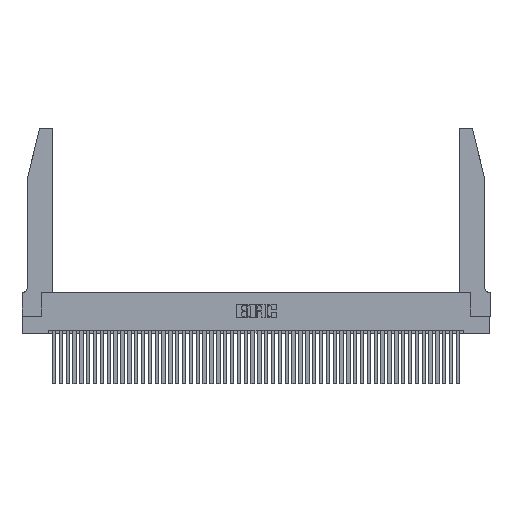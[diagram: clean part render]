
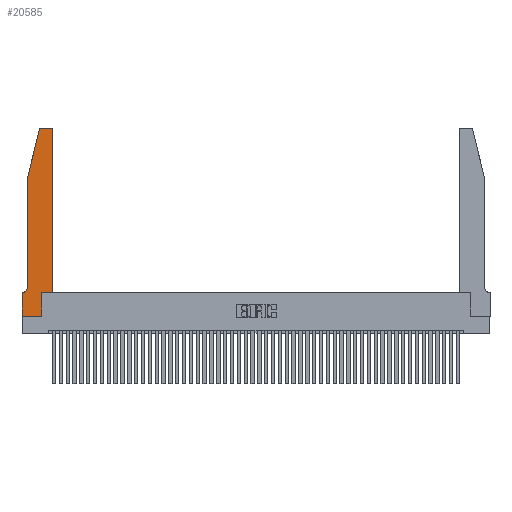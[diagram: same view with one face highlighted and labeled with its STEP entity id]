
A CAD part, top view. The second image highlights one B-rep face of the part: STEP entity #20585.
In plain terms, the highlighted planar face has unit normal (0, 0, 1).
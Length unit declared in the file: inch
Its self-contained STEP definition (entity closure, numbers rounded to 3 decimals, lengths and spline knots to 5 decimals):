
#116 = DIRECTION ( 'NONE',  ( 0., 0., 1. ) ) ;
#883 = CARTESIAN_POINT ( 'NONE',  ( 0.284, 2.72, 0.37 ) ) ;
#1681 = ORIENTED_EDGE ( 'NONE', *, *, #31914, .T. ) ;
#2662 = ORIENTED_EDGE ( 'NONE', *, *, #48983, .T. ) ;
#3055 = VERTEX_POINT ( 'NONE', #15933 ) ;
#3112 = EDGE_CURVE ( 'NONE', #3055, #36527, #25985, .T. ) ;
#3243 = DIRECTION ( 'NONE',  ( 0., 0., 1. ) ) ;
#5115 = CARTESIAN_POINT ( 'NONE',  ( 0.2865, 0.35, 0.37 ) ) ;
#5513 = CARTESIAN_POINT ( 'NONE',  ( 0.2865, 0.35, 0.37 ) ) ;
#5666 = DIRECTION ( 'NONE',  ( -0.239, -0.971, 0. ) ) ;
#7347 = CARTESIAN_POINT ( 'NONE',  ( 0.0055, 0.35, 0.37 ) ) ;
#8117 = CARTESIAN_POINT ( 'NONE',  ( 0.4205, 2.72, 0.37 ) ) ;
#8150 = VERTEX_POINT ( 'NONE', #7347 ) ;
#8230 = DIRECTION ( 'NONE',  ( 0., -1., 0. ) ) ;
#8537 = ORIENTED_EDGE ( 'NONE', *, *, #15006, .T. ) ;
#9021 = DIRECTION ( 'NONE',  ( 0., 0., 1. ) ) ;
#9081 = CARTESIAN_POINT ( 'NONE',  ( 0.0755, 2., 0.37 ) ) ;
#9732 = CARTESIAN_POINT ( 'NONE',  ( 0., 0., 0.37 ) ) ;
#12758 = AXIS2_PLACEMENT_3D ( 'NONE', #26011, #3243, #26318 ) ;
#13857 = VECTOR ( 'NONE', #45766, 39.37008 ) ;
#15006 = EDGE_CURVE ( 'NONE', #36527, #17993, #32076, .T. ) ;
#15134 = VECTOR ( 'NONE', #30617, 39.37008 ) ;
#15933 = CARTESIAN_POINT ( 'NONE',  ( 0.2865, 0., 0.37 ) ) ;
#16344 = DIRECTION ( 'NONE',  ( 1., 0., 0. ) ) ;
#16588 = ORIENTED_EDGE ( 'NONE', *, *, #36919, .T. ) ;
#16604 = DIRECTION ( 'NONE',  ( 0., 1., 0. ) ) ;
#17205 = CARTESIAN_POINT ( 'NONE',  ( 0.4505, 0.35, 0.37 ) ) ;
#17534 = DIRECTION ( 'NONE',  ( 0., 1., 0. ) ) ;
#17785 = AXIS2_PLACEMENT_3D ( 'NONE', #8117, #116, #23240 ) ;
#17876 = VECTOR ( 'NONE', #47383, 39.37008 ) ;
#17993 = VERTEX_POINT ( 'NONE', #24233 ) ;
#18170 = ORIENTED_EDGE ( 'NONE', *, *, #40487, .T. ) ;
#20585 = ADVANCED_FACE ( 'NONE', ( #42081 ), #22025, .T. ) ;
#20808 = CARTESIAN_POINT ( 'NONE',  ( 0.25487, 2.72718, 0.37 ) ) ;
#21279 = AXIS2_PLACEMENT_3D ( 'NONE', #25701, #25538, #21552 ) ;
#21552 = DIRECTION ( 'NONE',  ( -1., 0., 0. ) ) ;
#21608 = ORIENTED_EDGE ( 'NONE', *, *, #30950, .T. ) ;
#22025 = PLANE ( 'NONE',  #12758 ) ;
#22531 = CARTESIAN_POINT ( 'NONE',  ( 0., 0., 0.37 ) ) ;
#23240 = DIRECTION ( 'NONE',  ( 1., 0., 0. ) ) ;
#24166 = LINE ( 'NONE', #27849, #49148 ) ;
#24233 = CARTESIAN_POINT ( 'NONE',  ( 0.4505, 0.35, 0.37 ) ) ;
#24405 = ORIENTED_EDGE ( 'NONE', *, *, #43288, .T. ) ;
#24584 = ORIENTED_EDGE ( 'NONE', *, *, #38053, .T. ) ;
#24832 = VERTEX_POINT ( 'NONE', #42298 ) ;
#25123 = CIRCLE ( 'NONE', #21279, 0.07 ) ;
#25139 = EDGE_LOOP ( 'NONE', ( #1681, #2662, #18170, #30014, #21608, #16588, #49153, #24405, #34989, #8537, #24584, #27201 ) ) ;
#25298 = LINE ( 'NONE', #34484, #15134 ) ;
#25477 = LINE ( 'NONE', #47034, #49248 ) ;
#25538 = DIRECTION ( 'NONE',  ( 0., 0., -1. ) ) ;
#25701 = CARTESIAN_POINT ( 'NONE',  ( 0.0055, 0.42, 0.37 ) ) ;
#25963 = VERTEX_POINT ( 'NONE', #9081 ) ;
#25985 = LINE ( 'NONE', #5115, #30099 ) ;
#26011 = CARTESIAN_POINT ( 'NONE',  ( 0., 0.35, 0.37 ) ) ;
#26077 = VECTOR ( 'NONE', #40917, 39.37008 ) ;
#26318 = DIRECTION ( 'NONE',  ( 1., 0., 0. ) ) ;
#27201 = ORIENTED_EDGE ( 'NONE', *, *, #42684, .T. ) ;
#27849 = CARTESIAN_POINT ( 'NONE',  ( 0., 0., 0.37 ) ) ;
#27866 = CARTESIAN_POINT ( 'NONE',  ( 0., 0.35, 0.37 ) ) ;
#29054 = LINE ( 'NONE', #37125, #26077 ) ;
#29087 = VERTEX_POINT ( 'NONE', #30826 ) ;
#29121 = VECTOR ( 'NONE', #38011, 39.37008 ) ;
#29879 = VERTEX_POINT ( 'NONE', #46203 ) ;
#30014 = ORIENTED_EDGE ( 'NONE', *, *, #42051, .T. ) ;
#30099 = VECTOR ( 'NONE', #16604, 39.37008 ) ;
#30617 = DIRECTION ( 'NONE',  ( 0., -1., 0. ) ) ;
#30826 = CARTESIAN_POINT ( 'NONE',  ( 0.4205, 2.75, 0.37 ) ) ;
#30950 = EDGE_CURVE ( 'NONE', #37397, #8150, #25123, .T. ) ;
#31914 = EDGE_CURVE ( 'NONE', #29087, #29879, #41671, .T. ) ;
#32076 = LINE ( 'NONE', #45599, #29121 ) ;
#34239 = VERTEX_POINT ( 'NONE', #27866 ) ;
#34484 = CARTESIAN_POINT ( 'NONE',  ( 0.0755, 2., 0.37 ) ) ;
#34989 = ORIENTED_EDGE ( 'NONE', *, *, #3112, .T. ) ;
#36152 = LINE ( 'NONE', #17205, #39077 ) ;
#36527 = VERTEX_POINT ( 'NONE', #5513 ) ;
#36586 = CARTESIAN_POINT ( 'NONE',  ( 0.0755, 0.42, 0.37 ) ) ;
#36686 = CIRCLE ( 'NONE', #37317, 0.03 ) ;
#36919 = EDGE_CURVE ( 'NONE', #8150, #34239, #29054, .T. ) ;
#37125 = CARTESIAN_POINT ( 'NONE',  ( 0.0755, 0.35, 0.37 ) ) ;
#37317 = AXIS2_PLACEMENT_3D ( 'NONE', #883, #9021, #16344 ) ;
#37397 = VERTEX_POINT ( 'NONE', #36586 ) ;
#37800 = EDGE_CURVE ( 'NONE', #34239, #43003, #24166, .T. ) ;
#38011 = DIRECTION ( 'NONE',  ( 1., 0., 0. ) ) ;
#38053 = EDGE_CURVE ( 'NONE', #17993, #24832, #36152, .T. ) ;
#39077 = VECTOR ( 'NONE', #17534, 39.37008 ) ;
#40487 = EDGE_CURVE ( 'NONE', #44062, #25963, #25477, .T. ) ;
#40917 = DIRECTION ( 'NONE',  ( -1., 0., 0. ) ) ;
#41671 = LINE ( 'NONE', #47037, #17876 ) ;
#42051 = EDGE_CURVE ( 'NONE', #25963, #37397, #25298, .T. ) ;
#42081 = FACE_OUTER_BOUND ( 'NONE', #25139, .T. ) ;
#42298 = CARTESIAN_POINT ( 'NONE',  ( 0.4505, 2.72, 0.37 ) ) ;
#42684 = EDGE_CURVE ( 'NONE', #24832, #29087, #46627, .T. ) ;
#43003 = VERTEX_POINT ( 'NONE', #9732 ) ;
#43288 = EDGE_CURVE ( 'NONE', #43003, #3055, #44222, .T. ) ;
#44062 = VERTEX_POINT ( 'NONE', #20808 ) ;
#44222 = LINE ( 'NONE', #22531, #13857 ) ;
#45599 = CARTESIAN_POINT ( 'NONE',  ( 0.4505, 0.35, 0.37 ) ) ;
#45766 = DIRECTION ( 'NONE',  ( 1., 0., 0. ) ) ;
#46203 = CARTESIAN_POINT ( 'NONE',  ( 0.284, 2.75, 0.37 ) ) ;
#46627 = CIRCLE ( 'NONE', #17785, 0.03 ) ;
#47034 = CARTESIAN_POINT ( 'NONE',  ( 0.0755, 2., 0.37 ) ) ;
#47037 = CARTESIAN_POINT ( 'NONE',  ( 0.2605, 2.75, 0.37 ) ) ;
#47383 = DIRECTION ( 'NONE',  ( -1., 0., 0. ) ) ;
#48983 = EDGE_CURVE ( 'NONE', #29879, #44062, #36686, .T. ) ;
#49148 = VECTOR ( 'NONE', #8230, 39.37008 ) ;
#49153 = ORIENTED_EDGE ( 'NONE', *, *, #37800, .T. ) ;
#49248 = VECTOR ( 'NONE', #5666, 39.37008 ) ;
